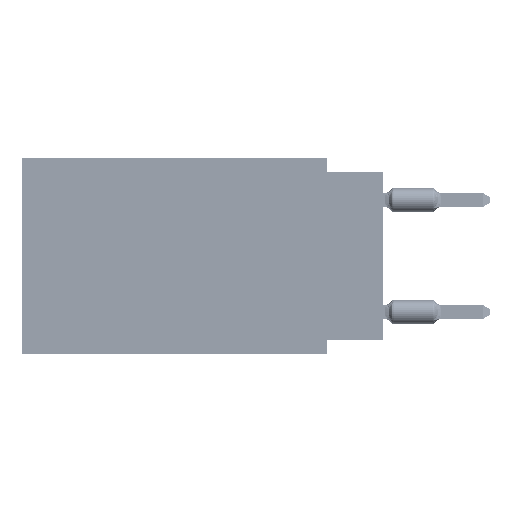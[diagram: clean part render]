
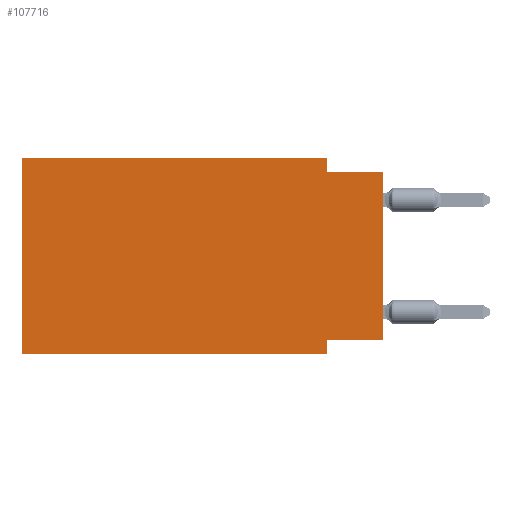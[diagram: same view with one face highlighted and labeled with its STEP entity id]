
A CAD part, left-side view. The second image highlights one B-rep face of the part: STEP entity #107716.
In plain terms, the highlighted planar face has unit normal (-1, 0, 0).
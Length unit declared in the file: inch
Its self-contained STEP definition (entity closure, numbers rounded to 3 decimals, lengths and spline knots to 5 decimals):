
#231 = CARTESIAN_POINT ( 'NONE',  ( 0., 0.1, 0. ) ) ;
#1721 = CARTESIAN_POINT ( 'NONE',  ( 0., 0.645, 0. ) ) ;
#2967 = ORIENTED_EDGE ( 'NONE', *, *, #17426, .T. ) ;
#5013 = VERTEX_POINT ( 'NONE', #19714 ) ;
#5866 = EDGE_CURVE ( 'NONE', #25008, #20020, #104909, .T. ) ;
#8134 = CARTESIAN_POINT ( 'NONE',  ( 0., 0.1, -0.35 ) ) ;
#8256 = EDGE_CURVE ( 'NONE', #37480, #5013, #74183, .T. ) ;
#9927 = LINE ( 'NONE', #77068, #45059 ) ;
#10545 = VERTEX_POINT ( 'NONE', #231 ) ;
#10589 = FACE_OUTER_BOUND ( 'NONE', #29651, .T. ) ;
#12172 = DIRECTION ( 'NONE',  ( 0., 0., 1. ) ) ;
#13231 = VECTOR ( 'NONE', #97142, 39.37008 ) ;
#15675 = VECTOR ( 'NONE', #12172, 39.37008 ) ;
#16606 = AXIS2_PLACEMENT_3D ( 'NONE', #1721, #35575, #102203 ) ;
#17256 = LINE ( 'NONE', #92759, #72336 ) ;
#17426 = EDGE_CURVE ( 'NONE', #84633, #42713, #21043, .T. ) ;
#17816 = PLANE ( 'NONE',  #16606 ) ;
#19714 = CARTESIAN_POINT ( 'NONE',  ( 0., 0.1, -0.35 ) ) ;
#20020 = VERTEX_POINT ( 'NONE', #47327 ) ;
#21043 = LINE ( 'NONE', #94927, #15675 ) ;
#24648 = CARTESIAN_POINT ( 'NONE',  ( 0., 0., -0.025 ) ) ;
#25008 = VERTEX_POINT ( 'NONE', #80384 ) ;
#26280 = CARTESIAN_POINT ( 'NONE',  ( 0., 0., -0.025 ) ) ;
#29407 = CARTESIAN_POINT ( 'NONE',  ( 0., 0., -0.325 ) ) ;
#29651 = EDGE_LOOP ( 'NONE', ( #2967, #97943, #101456, #35210, #39764, #39832, #73706, #90169 ) ) ;
#31341 = VERTEX_POINT ( 'NONE', #106970 ) ;
#34346 = DIRECTION ( 'NONE',  ( 0., -1., 0. ) ) ;
#35210 = ORIENTED_EDGE ( 'NONE', *, *, #97709, .F. ) ;
#35318 = CARTESIAN_POINT ( 'NONE',  ( 0., 0.1, 0. ) ) ;
#35575 = DIRECTION ( 'NONE',  ( 1., 0., 0. ) ) ;
#37480 = VERTEX_POINT ( 'NONE', #49809 ) ;
#39764 = ORIENTED_EDGE ( 'NONE', *, *, #5866, .F. ) ;
#39832 = ORIENTED_EDGE ( 'NONE', *, *, #108176, .T. ) ;
#41766 = VECTOR ( 'NONE', #91398, 39.37008 ) ;
#41792 = LINE ( 'NONE', #75630, #97956 ) ;
#42713 = VERTEX_POINT ( 'NONE', #24648 ) ;
#45059 = VECTOR ( 'NONE', #34346, 39.37008 ) ;
#47327 = CARTESIAN_POINT ( 'NONE',  ( 0., 0.645, 0. ) ) ;
#49809 = CARTESIAN_POINT ( 'NONE',  ( 0., 0.1, -0.325 ) ) ;
#50466 = EDGE_CURVE ( 'NONE', #31341, #42713, #102331, .T. ) ;
#50700 = DIRECTION ( 'NONE',  ( 0., -1., 0. ) ) ;
#54909 = CARTESIAN_POINT ( 'NONE',  ( 0., 0.645, 0. ) ) ;
#68608 = DIRECTION ( 'NONE',  ( 0., 0., -1. ) ) ;
#72336 = VECTOR ( 'NONE', #92210, 39.37008 ) ;
#73706 = ORIENTED_EDGE ( 'NONE', *, *, #8256, .F. ) ;
#74183 = LINE ( 'NONE', #8134, #41766 ) ;
#75630 = CARTESIAN_POINT ( 'NONE',  ( 0., 0., -0.325 ) ) ;
#77068 = CARTESIAN_POINT ( 'NONE',  ( 0., 0.645, -0.35 ) ) ;
#80384 = CARTESIAN_POINT ( 'NONE',  ( 0., 0.645, -0.35 ) ) ;
#84633 = VERTEX_POINT ( 'NONE', #29407 ) ;
#86021 = EDGE_CURVE ( 'NONE', #84633, #37480, #41792, .T. ) ;
#90169 = ORIENTED_EDGE ( 'NONE', *, *, #86021, .F. ) ;
#91398 = DIRECTION ( 'NONE',  ( 0., 0., -1. ) ) ;
#92210 = DIRECTION ( 'NONE',  ( 0., -1., 0. ) ) ;
#92759 = CARTESIAN_POINT ( 'NONE',  ( 0., 0.645, 0. ) ) ;
#94927 = CARTESIAN_POINT ( 'NONE',  ( 0., 0., 0. ) ) ;
#97142 = DIRECTION ( 'NONE',  ( 0., 0., 1. ) ) ;
#97709 = EDGE_CURVE ( 'NONE', #20020, #10545, #17256, .T. ) ;
#97943 = ORIENTED_EDGE ( 'NONE', *, *, #50466, .F. ) ;
#97956 = VECTOR ( 'NONE', #100081, 39.37008 ) ;
#100081 = DIRECTION ( 'NONE',  ( 0., 1., 0. ) ) ;
#100405 = VECTOR ( 'NONE', #50700, 39.37008 ) ;
#101456 = ORIENTED_EDGE ( 'NONE', *, *, #108539, .F. ) ;
#101806 = VECTOR ( 'NONE', #68608, 39.37008 ) ;
#101947 = LINE ( 'NONE', #35318, #101806 ) ;
#102203 = DIRECTION ( 'NONE',  ( 0., 0., -1. ) ) ;
#102331 = LINE ( 'NONE', #26280, #100405 ) ;
#104909 = LINE ( 'NONE', #54909, #13231 ) ;
#106970 = CARTESIAN_POINT ( 'NONE',  ( 0., 0.1, -0.025 ) ) ;
#107716 = ADVANCED_FACE ( 'NONE', ( #10589 ), #17816, .F. ) ;
#108176 = EDGE_CURVE ( 'NONE', #25008, #5013, #9927, .T. ) ;
#108539 = EDGE_CURVE ( 'NONE', #10545, #31341, #101947, .T. ) ;
